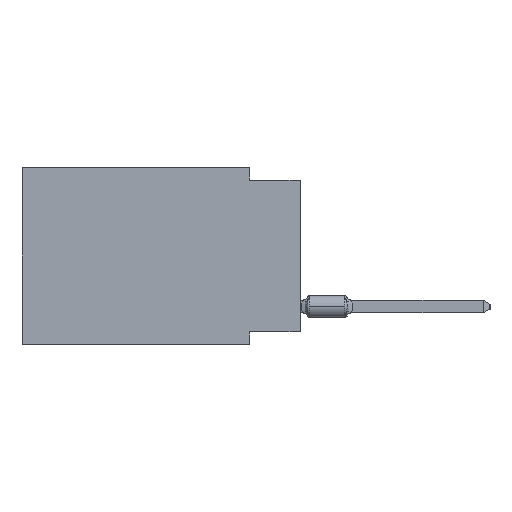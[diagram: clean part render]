
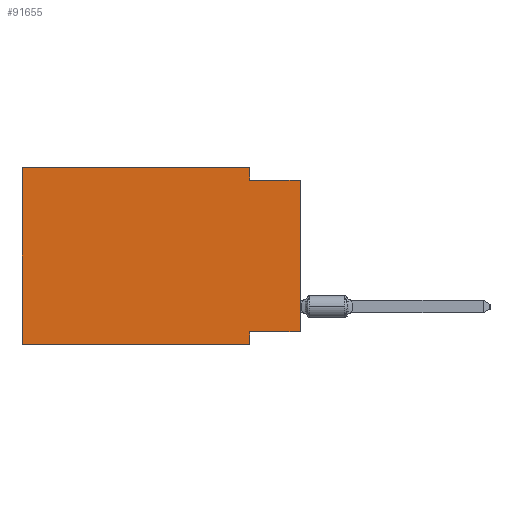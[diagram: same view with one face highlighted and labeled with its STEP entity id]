
A CAD part, left-side view. The second image highlights one B-rep face of the part: STEP entity #91655.
In plain terms, the highlighted planar face has unit normal (-1, 0, 0).
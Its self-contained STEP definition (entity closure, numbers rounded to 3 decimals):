
#556 = DIRECTION ( 'NONE',  ( 0., -1., 0. ) ) ;
#2874 = PLANE ( 'NONE',  #106367 ) ;
#4510 = VERTEX_POINT ( 'NONE', #110559 ) ;
#6160 = CARTESIAN_POINT ( 'NONE',  ( 0., 0., -8.255 ) ) ;
#9432 = CARTESIAN_POINT ( 'NONE',  ( 0., 0., 0. ) ) ;
#9704 = CARTESIAN_POINT ( 'NONE',  ( 0., 2.54, -0.635 ) ) ;
#10525 = ORIENTED_EDGE ( 'NONE', *, *, #70884, .F. ) ;
#11310 = LINE ( 'NONE', #103026, #72558 ) ;
#11531 = EDGE_CURVE ( 'NONE', #48329, #37344, #36834, .T. ) ;
#12978 = FACE_OUTER_BOUND ( 'NONE', #37336, .T. ) ;
#13668 = DIRECTION ( 'NONE',  ( 0., -1., 0. ) ) ;
#13764 = LINE ( 'NONE', #40583, #56038 ) ;
#15192 = CARTESIAN_POINT ( 'NONE',  ( 0., 0., -0.635 ) ) ;
#19398 = EDGE_CURVE ( 'NONE', #84261, #4510, #11310, .T. ) ;
#22205 = EDGE_CURVE ( 'NONE', #4510, #93644, #104220, .T. ) ;
#27245 = DIRECTION ( 'NONE',  ( 0., 0., -1. ) ) ;
#28933 = VECTOR ( 'NONE', #556, 1000. ) ;
#29660 = DIRECTION ( 'NONE',  ( 0., 0., 1. ) ) ;
#32150 = DIRECTION ( 'NONE',  ( 0., 0., -1. ) ) ;
#32190 = ORIENTED_EDGE ( 'NONE', *, *, #90200, .F. ) ;
#32227 = DIRECTION ( 'NONE',  ( 0., -1., 0. ) ) ;
#33785 = VERTEX_POINT ( 'NONE', #9704 ) ;
#35591 = CARTESIAN_POINT ( 'NONE',  ( 0., 2.54, -8.89 ) ) ;
#35812 = CARTESIAN_POINT ( 'NONE',  ( 0., 2.54, -8.89 ) ) ;
#36470 = CARTESIAN_POINT ( 'NONE',  ( 0., 0., -8.255 ) ) ;
#36834 = LINE ( 'NONE', #9432, #103618 ) ;
#37336 = EDGE_LOOP ( 'NONE', ( #77800, #95401, #32190, #57804, #109141, #48444, #10525, #67431 ) ) ;
#37344 = VERTEX_POINT ( 'NONE', #15192 ) ;
#39986 = EDGE_CURVE ( 'NONE', #84261, #58585, #13764, .T. ) ;
#40583 = CARTESIAN_POINT ( 'NONE',  ( 0., 13.97, -8.89 ) ) ;
#42152 = VERTEX_POINT ( 'NONE', #77079 ) ;
#45826 = CARTESIAN_POINT ( 'NONE',  ( 0., 2.54, 0. ) ) ;
#46985 = DIRECTION ( 'NONE',  ( 1., 0., 0. ) ) ;
#48329 = VERTEX_POINT ( 'NONE', #6160 ) ;
#48444 = ORIENTED_EDGE ( 'NONE', *, *, #39986, .T. ) ;
#49454 = LINE ( 'NONE', #67900, #115187 ) ;
#56038 = VECTOR ( 'NONE', #32227, 1000. ) ;
#56510 = CARTESIAN_POINT ( 'NONE',  ( 0., 13.97, 0. ) ) ;
#57189 = CARTESIAN_POINT ( 'NONE',  ( 0., 13.97, 0. ) ) ;
#57804 = ORIENTED_EDGE ( 'NONE', *, *, #22205, .F. ) ;
#58585 = VERTEX_POINT ( 'NONE', #35812 ) ;
#60756 = VECTOR ( 'NONE', #27245, 1000. ) ;
#61353 = EDGE_CURVE ( 'NONE', #33785, #37344, #98850, .T. ) ;
#62086 = LINE ( 'NONE', #36470, #110253 ) ;
#63828 = VECTOR ( 'NONE', #13668, 1000. ) ;
#64860 = CARTESIAN_POINT ( 'NONE',  ( 0., 0., -0.635 ) ) ;
#67431 = ORIENTED_EDGE ( 'NONE', *, *, #113028, .F. ) ;
#67900 = CARTESIAN_POINT ( 'NONE',  ( 0., 2.54, 0. ) ) ;
#70884 = EDGE_CURVE ( 'NONE', #42152, #58585, #73089, .T. ) ;
#71625 = DIRECTION ( 'NONE',  ( 0., 1., 0. ) ) ;
#72558 = VECTOR ( 'NONE', #113126, 1000. ) ;
#73089 = LINE ( 'NONE', #35591, #60756 ) ;
#73661 = CARTESIAN_POINT ( 'NONE',  ( 0., 13.97, -8.89 ) ) ;
#74937 = DIRECTION ( 'NONE',  ( 0., 0., -1. ) ) ;
#77079 = CARTESIAN_POINT ( 'NONE',  ( 0., 2.54, -8.255 ) ) ;
#77800 = ORIENTED_EDGE ( 'NONE', *, *, #11531, .T. ) ;
#84261 = VERTEX_POINT ( 'NONE', #73661 ) ;
#90200 = EDGE_CURVE ( 'NONE', #93644, #33785, #49454, .T. ) ;
#91655 = ADVANCED_FACE ( 'NONE', ( #12978 ), #2874, .F. ) ;
#93644 = VERTEX_POINT ( 'NONE', #45826 ) ;
#95401 = ORIENTED_EDGE ( 'NONE', *, *, #61353, .F. ) ;
#98850 = LINE ( 'NONE', #64860, #28933 ) ;
#103026 = CARTESIAN_POINT ( 'NONE',  ( 0., 13.97, 0. ) ) ;
#103618 = VECTOR ( 'NONE', #29660, 1000. ) ;
#104220 = LINE ( 'NONE', #57189, #63828 ) ;
#106367 = AXIS2_PLACEMENT_3D ( 'NONE', #56510, #46985, #74937 ) ;
#109141 = ORIENTED_EDGE ( 'NONE', *, *, #19398, .F. ) ;
#110253 = VECTOR ( 'NONE', #71625, 1000. ) ;
#110559 = CARTESIAN_POINT ( 'NONE',  ( 0., 13.97, 0. ) ) ;
#113028 = EDGE_CURVE ( 'NONE', #48329, #42152, #62086, .T. ) ;
#113126 = DIRECTION ( 'NONE',  ( 0., 0., 1. ) ) ;
#115187 = VECTOR ( 'NONE', #32150, 1000. ) ;
